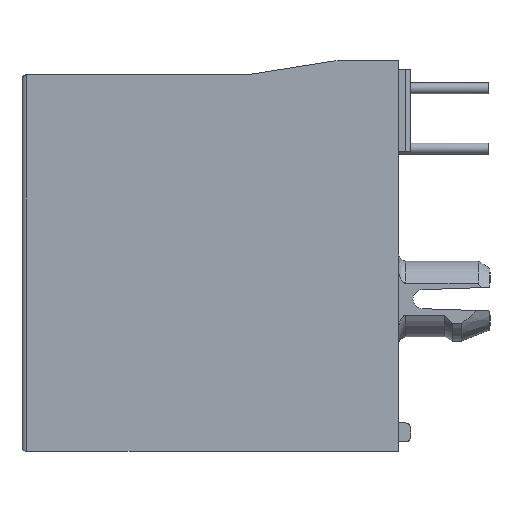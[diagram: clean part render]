
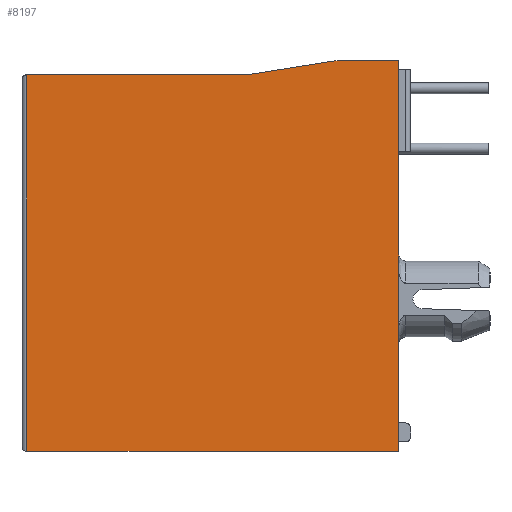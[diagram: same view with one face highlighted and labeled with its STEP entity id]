
A CAD part, left-side view. The second image highlights one B-rep face of the part: STEP entity #8197.
In plain terms, the highlighted planar face has unit normal (-1, 0, 0).
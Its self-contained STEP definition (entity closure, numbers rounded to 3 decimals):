
#571 = EDGE_CURVE ( 'NONE', #2625, #5088, #8399, .T. ) ;
#1169 = CARTESIAN_POINT ( 'NONE',  ( -6.73, -1.525, 9.46 ) ) ;
#1309 = DIRECTION ( 'NONE',  ( 0., 0., -1. ) ) ;
#1544 = VECTOR ( 'NONE', #7208, 1000. ) ;
#1619 = VECTOR ( 'NONE', #10014, 1000. ) ;
#2175 = EDGE_CURVE ( 'NONE', #13442, #13663, #10401, .T. ) ;
#2625 = VERTEX_POINT ( 'NONE', #1169 ) ;
#3017 = DIRECTION ( 'NONE',  ( 0., 0., 1. ) ) ;
#3479 = LINE ( 'NONE', #6678, #9881 ) ;
#3891 = LINE ( 'NONE', #7366, #7642 ) ;
#4054 = ORIENTED_EDGE ( 'NONE', *, *, #2175, .T. ) ;
#4066 = ORIENTED_EDGE ( 'NONE', *, *, #11089, .T. ) ;
#5088 = VERTEX_POINT ( 'NONE', #13913 ) ;
#5116 = VECTOR ( 'NONE', #5625, 1000. ) ;
#5607 = ORIENTED_EDGE ( 'NONE', *, *, #5804, .T. ) ;
#5625 = DIRECTION ( 'NONE',  ( 0., 1., 0. ) ) ;
#5660 = CARTESIAN_POINT ( 'NONE',  ( -6.73, -5.305, 10.06 ) ) ;
#5804 = EDGE_CURVE ( 'NONE', #13663, #2625, #12250, .T. ) ;
#5918 = DIRECTION ( 'NONE',  ( 0., -1., 0. ) ) ;
#6678 = CARTESIAN_POINT ( 'NONE',  ( -6.73, -7.905, 1.82 ) ) ;
#7165 = CARTESIAN_POINT ( 'NONE',  ( -6.73, -7.905, -6.42 ) ) ;
#7208 = DIRECTION ( 'NONE',  ( 0., 0.988, -0.157 ) ) ;
#7366 = CARTESIAN_POINT ( 'NONE',  ( -6.73, 7.775, 1.82 ) ) ;
#7548 = AXIS2_PLACEMENT_3D ( 'NONE', #10338, #7654, #14070 ) ;
#7609 = ORIENTED_EDGE ( 'NONE', *, *, #571, .T. ) ;
#7642 = VECTOR ( 'NONE', #1309, 1000. ) ;
#7654 = DIRECTION ( 'NONE',  ( -1., 0., 0. ) ) ;
#8197 = ADVANCED_FACE ( 'NONE', ( #14428 ), #14793, .T. ) ;
#8399 = LINE ( 'NONE', #12483, #1619 ) ;
#8569 = EDGE_CURVE ( 'NONE', #5088, #9175, #3891, .T. ) ;
#9175 = VERTEX_POINT ( 'NONE', #10554 ) ;
#9881 = VECTOR ( 'NONE', #3017, 1000. ) ;
#9933 = ORIENTED_EDGE ( 'NONE', *, *, #8569, .T. ) ;
#10014 = DIRECTION ( 'NONE',  ( 0., 1., 0. ) ) ;
#10338 = CARTESIAN_POINT ( 'NONE',  ( -6.73, 0.035, 1.82 ) ) ;
#10401 = LINE ( 'NONE', #15273, #5116 ) ;
#10554 = CARTESIAN_POINT ( 'NONE',  ( -6.73, 7.775, -6.42 ) ) ;
#10693 = CARTESIAN_POINT ( 'NONE',  ( -6.73, -5.305, 10.06 ) ) ;
#11089 = EDGE_CURVE ( 'NONE', #14109, #13442, #3479, .T. ) ;
#12250 = LINE ( 'NONE', #10693, #1544 ) ;
#12283 = ORIENTED_EDGE ( 'NONE', *, *, #15081, .T. ) ;
#12476 = CARTESIAN_POINT ( 'NONE',  ( -6.73, -7.905, 10.06 ) ) ;
#12483 = CARTESIAN_POINT ( 'NONE',  ( -6.73, 0.035, 9.46 ) ) ;
#12591 = LINE ( 'NONE', #13090, #15230 ) ;
#13090 = CARTESIAN_POINT ( 'NONE',  ( -6.73, 0.035, -6.42 ) ) ;
#13294 = EDGE_LOOP ( 'NONE', ( #12283, #4066, #4054, #5607, #7609, #9933 ) ) ;
#13442 = VERTEX_POINT ( 'NONE', #12476 ) ;
#13663 = VERTEX_POINT ( 'NONE', #5660 ) ;
#13913 = CARTESIAN_POINT ( 'NONE',  ( -6.73, 7.775, 9.46 ) ) ;
#14070 = DIRECTION ( 'NONE',  ( 0., 0., 1. ) ) ;
#14109 = VERTEX_POINT ( 'NONE', #7165 ) ;
#14428 = FACE_OUTER_BOUND ( 'NONE', #13294, .T. ) ;
#14793 = PLANE ( 'NONE',  #7548 ) ;
#15081 = EDGE_CURVE ( 'NONE', #9175, #14109, #12591, .T. ) ;
#15230 = VECTOR ( 'NONE', #5918, 1000. ) ;
#15273 = CARTESIAN_POINT ( 'NONE',  ( -6.73, 0.035, 10.06 ) ) ;
